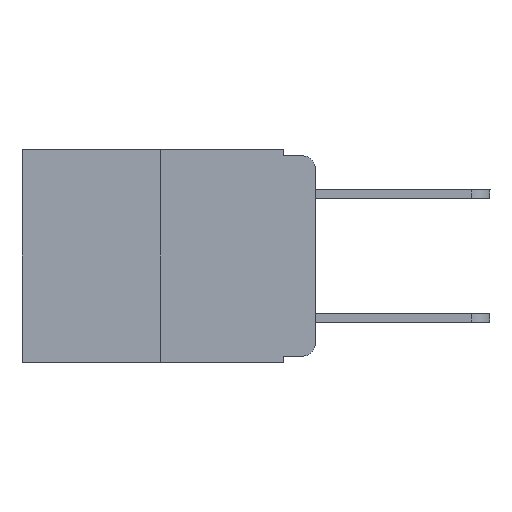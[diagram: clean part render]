
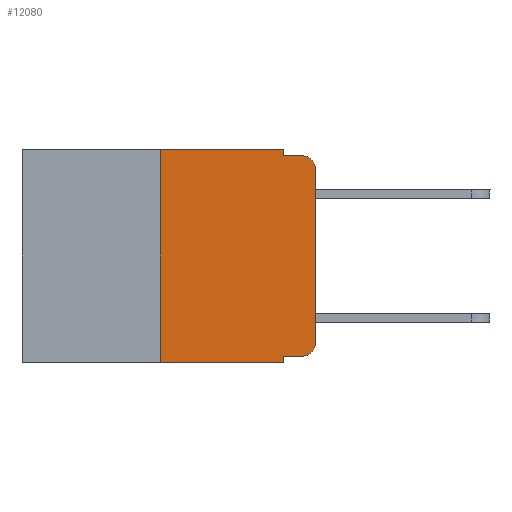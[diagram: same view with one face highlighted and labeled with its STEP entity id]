
A CAD part, left-side view. The second image highlights one B-rep face of the part: STEP entity #12080.
In plain terms, the highlighted planar face has unit normal (-1, 0, 0).
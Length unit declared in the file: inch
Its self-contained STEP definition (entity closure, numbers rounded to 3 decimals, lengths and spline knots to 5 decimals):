
#59 = LINE ( 'NONE', #4877, #2729 ) ;
#199 = CARTESIAN_POINT ( 'NONE',  ( 0., 0.473, 0. ) ) ;
#291 = ORIENTED_EDGE ( 'NONE', *, *, #14071, .T. ) ;
#295 = VECTOR ( 'NONE', #4230, 39.37008 ) ;
#406 = EDGE_CURVE ( 'NONE', #7150, #14961, #5527, .T. ) ;
#652 = DIRECTION ( 'NONE',  ( 0., -1., 0. ) ) ;
#733 = CARTESIAN_POINT ( 'NONE',  ( 0., 0.051, -0.333 ) ) ;
#981 = VECTOR ( 'NONE', #9386, 39.37008 ) ;
#1109 = ORIENTED_EDGE ( 'NONE', *, *, #14671, .T. ) ;
#1264 = ORIENTED_EDGE ( 'NONE', *, *, #15137, .F. ) ;
#1413 = DIRECTION ( 'NONE',  ( 0., 0., -1. ) ) ;
#1527 = DIRECTION ( 'NONE',  ( 0., 0., -1. ) ) ;
#1556 = VERTEX_POINT ( 'NONE', #13201 ) ;
#1939 = VERTEX_POINT ( 'NONE', #2851 ) ;
#2199 = EDGE_CURVE ( 'NONE', #13948, #2618, #9529, .T. ) ;
#2230 = VERTEX_POINT ( 'NONE', #7351 ) ;
#2508 = VECTOR ( 'NONE', #1527, 39.37008 ) ;
#2618 = VERTEX_POINT ( 'NONE', #13279 ) ;
#2729 = VECTOR ( 'NONE', #8734, 39.37008 ) ;
#2851 = CARTESIAN_POINT ( 'NONE',  ( 0., 0.02, -0.01 ) ) ;
#3147 = ORIENTED_EDGE ( 'NONE', *, *, #2199, .F. ) ;
#3578 = LINE ( 'NONE', #4460, #981 ) ;
#3592 = DIRECTION ( 'NONE',  ( -1., 0., 0. ) ) ;
#3603 = VECTOR ( 'NONE', #9627, 39.37008 ) ;
#3604 = AXIS2_PLACEMENT_3D ( 'NONE', #12296, #3592, #1413 ) ;
#3613 = EDGE_CURVE ( 'NONE', #2230, #11494, #13852, .T. ) ;
#3823 = VECTOR ( 'NONE', #12255, 39.37008 ) ;
#3920 = CARTESIAN_POINT ( 'NONE',  ( 0., 0., -0.313 ) ) ;
#4230 = DIRECTION ( 'NONE',  ( 0., 0., -1. ) ) ;
#4460 = CARTESIAN_POINT ( 'NONE',  ( 0., 0.473, -0.343 ) ) ;
#4495 = CARTESIAN_POINT ( 'NONE',  ( 0., 0.051, -0.343 ) ) ;
#4566 = CARTESIAN_POINT ( 'NONE',  ( 0., 0.051, 0. ) ) ;
#4585 = CARTESIAN_POINT ( 'NONE',  ( 0., 0.051, -0.01 ) ) ;
#4877 = CARTESIAN_POINT ( 'NONE',  ( 0., 0.473, 0. ) ) ;
#4906 = VECTOR ( 'NONE', #652, 39.37008 ) ;
#5406 = CIRCLE ( 'NONE', #3604, 0.02 ) ;
#5527 = CIRCLE ( 'NONE', #5770, 0.02 ) ;
#5604 = DIRECTION ( 'NONE',  ( -1., 0., 0. ) ) ;
#5770 = AXIS2_PLACEMENT_3D ( 'NONE', #10742, #5604, #9384 ) ;
#6167 = FACE_OUTER_BOUND ( 'NONE', #6287, .T. ) ;
#6287 = EDGE_LOOP ( 'NONE', ( #12229, #291, #12468, #1264, #10083, #3147, #10912, #10406, #1109, #15302 ) ) ;
#6904 = CARTESIAN_POINT ( 'NONE',  ( 0., 0.25, -0.343 ) ) ;
#7150 = VERTEX_POINT ( 'NONE', #15515 ) ;
#7351 = CARTESIAN_POINT ( 'NONE',  ( 0., 0.051, -0.333 ) ) ;
#7696 = VECTOR ( 'NONE', #14438, 39.37008 ) ;
#8194 = AXIS2_PLACEMENT_3D ( 'NONE', #199, #13479, #14838 ) ;
#8322 = CARTESIAN_POINT ( 'NONE',  ( 0., 0.25, 0. ) ) ;
#8734 = DIRECTION ( 'NONE',  ( 0., -1., 0. ) ) ;
#9112 = CARTESIAN_POINT ( 'NONE',  ( 0., 0.051, 0. ) ) ;
#9384 = DIRECTION ( 'NONE',  ( 0., 0., -1. ) ) ;
#9386 = DIRECTION ( 'NONE',  ( 0., -1., 0. ) ) ;
#9529 = LINE ( 'NONE', #8322, #7696 ) ;
#9627 = DIRECTION ( 'NONE',  ( 0., -1., 0. ) ) ;
#10083 = ORIENTED_EDGE ( 'NONE', *, *, #10350, .F. ) ;
#10156 = LINE ( 'NONE', #733, #4906 ) ;
#10350 = EDGE_CURVE ( 'NONE', #2618, #15291, #59, .T. ) ;
#10406 = ORIENTED_EDGE ( 'NONE', *, *, #3613, .F. ) ;
#10742 = CARTESIAN_POINT ( 'NONE',  ( 0., 0.02, -0.313 ) ) ;
#10752 = LINE ( 'NONE', #15658, #3603 ) ;
#10912 = ORIENTED_EDGE ( 'NONE', *, *, #11971, .T. ) ;
#11065 = PLANE ( 'NONE',  #8194 ) ;
#11494 = VERTEX_POINT ( 'NONE', #4495 ) ;
#11971 = EDGE_CURVE ( 'NONE', #13948, #11494, #3578, .T. ) ;
#12080 = ADVANCED_FACE ( 'NONE', ( #6167 ), #11065, .F. ) ;
#12229 = ORIENTED_EDGE ( 'NONE', *, *, #12473, .T. ) ;
#12255 = DIRECTION ( 'NONE',  ( 0., 0., 1. ) ) ;
#12296 = CARTESIAN_POINT ( 'NONE',  ( 0., 0.02, -0.03 ) ) ;
#12468 = ORIENTED_EDGE ( 'NONE', *, *, #15723, .F. ) ;
#12473 = EDGE_CURVE ( 'NONE', #14961, #1556, #13377, .T. ) ;
#13201 = CARTESIAN_POINT ( 'NONE',  ( 0., 0., -0.03 ) ) ;
#13279 = CARTESIAN_POINT ( 'NONE',  ( 0., 0.25, 0. ) ) ;
#13377 = LINE ( 'NONE', #15872, #3823 ) ;
#13479 = DIRECTION ( 'NONE',  ( 1., 0., 0. ) ) ;
#13852 = LINE ( 'NONE', #9112, #2508 ) ;
#13948 = VERTEX_POINT ( 'NONE', #6904 ) ;
#13981 = CARTESIAN_POINT ( 'NONE',  ( 0., 0.051, 0. ) ) ;
#14060 = LINE ( 'NONE', #13981, #295 ) ;
#14071 = EDGE_CURVE ( 'NONE', #1556, #1939, #5406, .T. ) ;
#14438 = DIRECTION ( 'NONE',  ( 0., 0., 1. ) ) ;
#14671 = EDGE_CURVE ( 'NONE', #2230, #7150, #10156, .T. ) ;
#14826 = VERTEX_POINT ( 'NONE', #4585 ) ;
#14838 = DIRECTION ( 'NONE',  ( 0., 0., -1. ) ) ;
#14961 = VERTEX_POINT ( 'NONE', #3920 ) ;
#15137 = EDGE_CURVE ( 'NONE', #15291, #14826, #14060, .T. ) ;
#15291 = VERTEX_POINT ( 'NONE', #4566 ) ;
#15302 = ORIENTED_EDGE ( 'NONE', *, *, #406, .T. ) ;
#15515 = CARTESIAN_POINT ( 'NONE',  ( 0., 0.02, -0.333 ) ) ;
#15658 = CARTESIAN_POINT ( 'NONE',  ( 0., 0.051, -0.01 ) ) ;
#15723 = EDGE_CURVE ( 'NONE', #14826, #1939, #10752, .T. ) ;
#15872 = CARTESIAN_POINT ( 'NONE',  ( 0., 0., 0. ) ) ;
